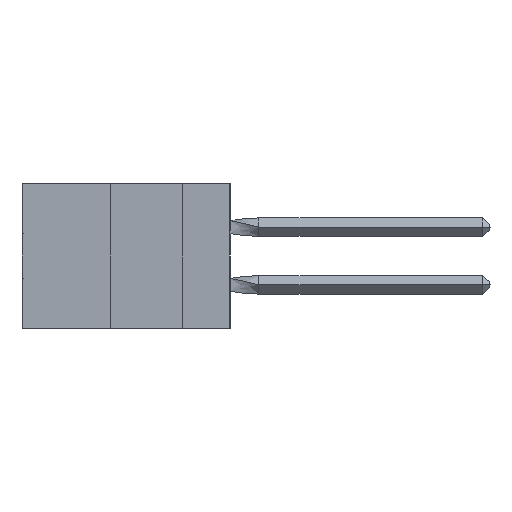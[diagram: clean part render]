
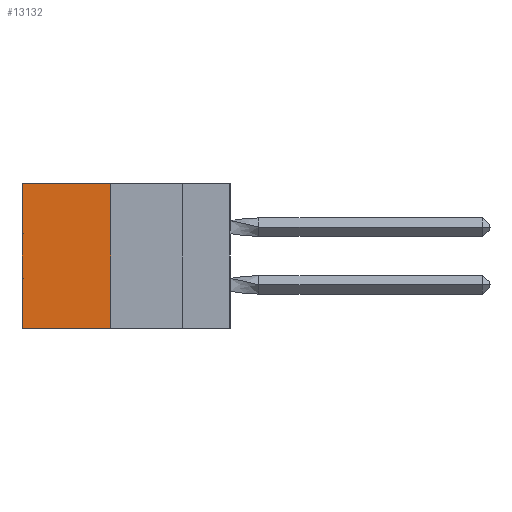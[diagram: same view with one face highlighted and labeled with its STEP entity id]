
A CAD part, left-side view. The second image highlights one B-rep face of the part: STEP entity #13132.
In plain terms, the highlighted planar face has unit normal (-1, 0, 0).
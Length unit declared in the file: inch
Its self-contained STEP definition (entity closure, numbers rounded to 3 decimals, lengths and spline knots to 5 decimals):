
#1639 = VECTOR ( 'NONE', #12115, 39.37008 ) ;
#1968 = ORIENTED_EDGE ( 'NONE', *, *, #41253, .T. ) ;
#3288 = VERTEX_POINT ( 'NONE', #6874 ) ;
#4452 = DIRECTION ( 'NONE',  ( 0., 1., 0. ) ) ;
#5286 = LINE ( 'NONE', #31963, #22199 ) ;
#5357 = ORIENTED_EDGE ( 'NONE', *, *, #17004, .F. ) ;
#6754 = VERTEX_POINT ( 'NONE', #44638 ) ;
#6874 = CARTESIAN_POINT ( 'NONE',  ( 0.305, 0.72, 0. ) ) ;
#7021 = PLANE ( 'NONE',  #29615 ) ;
#9006 = EDGE_CURVE ( 'NONE', #6754, #35195, #30815, .T. ) ;
#11329 = LINE ( 'NONE', #19919, #1639 ) ;
#12115 = DIRECTION ( 'NONE',  ( 0., 1., 0. ) ) ;
#12754 = DIRECTION ( 'NONE',  ( 0., 0., -1. ) ) ;
#13132 = ADVANCED_FACE ( 'NONE', ( #22655 ), #7021, .F. ) ;
#13934 = DIRECTION ( 'NONE',  ( 0., 0., -1. ) ) ;
#14602 = ORIENTED_EDGE ( 'NONE', *, *, #16081, .T. ) ;
#16081 = EDGE_CURVE ( 'NONE', #6754, #3288, #50079, .T. ) ;
#16372 = VECTOR ( 'NONE', #13934, 39.37008 ) ;
#17004 = EDGE_CURVE ( 'NONE', #35195, #45469, #11329, .T. ) ;
#17997 = CARTESIAN_POINT ( 'NONE',  ( 0.305, 0.72, -0.5 ) ) ;
#19119 = CARTESIAN_POINT ( 'NONE',  ( 0.305, 0.413, 0. ) ) ;
#19919 = CARTESIAN_POINT ( 'NONE',  ( 0.305, 0.413, -0.5 ) ) ;
#22131 = CARTESIAN_POINT ( 'NONE',  ( 0.305, 0.413, -0.5 ) ) ;
#22199 = VECTOR ( 'NONE', #12754, 39.37008 ) ;
#22655 = FACE_OUTER_BOUND ( 'NONE', #23269, .T. ) ;
#22726 = ORIENTED_EDGE ( 'NONE', *, *, #9006, .F. ) ;
#23269 = EDGE_LOOP ( 'NONE', ( #1968, #5357, #22726, #14602 ) ) ;
#28894 = VECTOR ( 'NONE', #4452, 39.37008 ) ;
#29615 = AXIS2_PLACEMENT_3D ( 'NONE', #42830, #31592, #43391 ) ;
#30815 = LINE ( 'NONE', #22131, #16372 ) ;
#31592 = DIRECTION ( 'NONE',  ( 1., 0., 0. ) ) ;
#31963 = CARTESIAN_POINT ( 'NONE',  ( 0.305, 0.72, -0.5 ) ) ;
#35195 = VERTEX_POINT ( 'NONE', #45522 ) ;
#41253 = EDGE_CURVE ( 'NONE', #3288, #45469, #5286, .T. ) ;
#42830 = CARTESIAN_POINT ( 'NONE',  ( 0.305, 0.413, -0.5 ) ) ;
#43391 = DIRECTION ( 'NONE',  ( 0., 0., -1. ) ) ;
#44638 = CARTESIAN_POINT ( 'NONE',  ( 0.305, 0.413, 0. ) ) ;
#45469 = VERTEX_POINT ( 'NONE', #17997 ) ;
#45522 = CARTESIAN_POINT ( 'NONE',  ( 0.305, 0.413, -0.5 ) ) ;
#50079 = LINE ( 'NONE', #19119, #28894 ) ;
